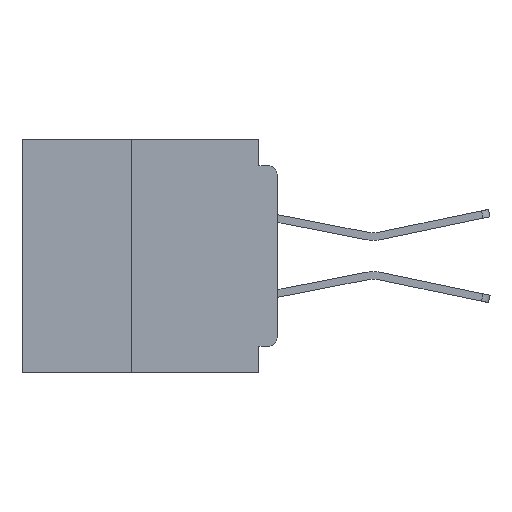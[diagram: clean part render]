
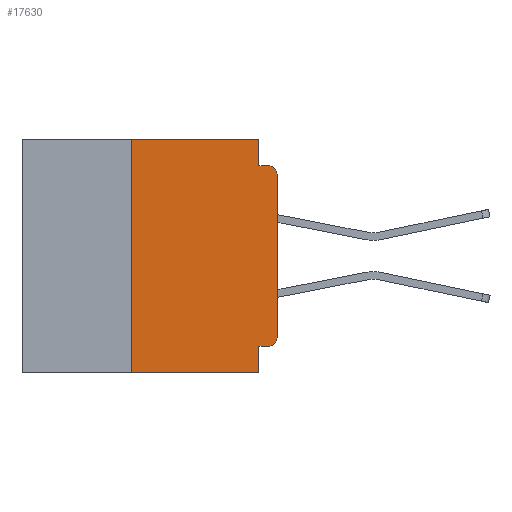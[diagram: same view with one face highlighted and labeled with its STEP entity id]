
A CAD part, left-side view. The second image highlights one B-rep face of the part: STEP entity #17630.
In plain terms, the highlighted planar face has unit normal (-1, 0, 0).
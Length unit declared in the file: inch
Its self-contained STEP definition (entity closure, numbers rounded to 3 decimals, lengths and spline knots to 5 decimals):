
#863 = VERTEX_POINT ( 'NONE', #28251 ) ;
#1961 = VERTEX_POINT ( 'NONE', #22788 ) ;
#3124 = DIRECTION ( 'NONE',  ( 0., -1., 0. ) ) ;
#4125 = DIRECTION ( 'NONE',  ( 0., 0., 1. ) ) ;
#4269 = DIRECTION ( 'NONE',  ( 0., -1., 0. ) ) ;
#4280 = ORIENTED_EDGE ( 'NONE', *, *, #34352, .F. ) ;
#4427 = VECTOR ( 'NONE', #4125, 39.37008 ) ;
#4716 = EDGE_CURVE ( 'NONE', #42640, #46882, #25046, .T. ) ;
#4944 = LINE ( 'NONE', #31945, #31008 ) ;
#5042 = DIRECTION ( 'NONE',  ( 0., 1., 0. ) ) ;
#5555 = CARTESIAN_POINT ( 'NONE',  ( 0., 0.031, -0.4 ) ) ;
#5792 = LINE ( 'NONE', #15640, #31858 ) ;
#5839 = CARTESIAN_POINT ( 'NONE',  ( 0., 0.015, -0.355 ) ) ;
#6506 = DIRECTION ( 'NONE',  ( -1., 0., 0. ) ) ;
#6541 = DIRECTION ( 'NONE',  ( 0., 0., 1. ) ) ;
#8428 = VERTEX_POINT ( 'NONE', #54226 ) ;
#10193 = DIRECTION ( 'NONE',  ( 0., 0., -1. ) ) ;
#10195 = CARTESIAN_POINT ( 'NONE',  ( 0., 0., -0.06 ) ) ;
#10734 = PLANE ( 'NONE',  #24280 ) ;
#11430 = EDGE_LOOP ( 'NONE', ( #28091, #58225, #35325, #39648, #4280, #16560, #43976, #33173, #38935, #40391 ) ) ;
#11553 = AXIS2_PLACEMENT_3D ( 'NONE', #34167, #6506, #38782 ) ;
#13358 = EDGE_CURVE ( 'NONE', #1961, #33585, #40653, .T. ) ;
#14480 = LINE ( 'NONE', #23414, #49854 ) ;
#15387 = DIRECTION ( 'NONE',  ( 1., 0., 0. ) ) ;
#15640 = CARTESIAN_POINT ( 'NONE',  ( 0., 0.25, -0.4 ) ) ;
#16560 = ORIENTED_EDGE ( 'NONE', *, *, #54841, .F. ) ;
#17630 = ADVANCED_FACE ( 'NONE', ( #53106 ), #10734, .F. ) ;
#18800 = VERTEX_POINT ( 'NONE', #10195 ) ;
#21781 = CARTESIAN_POINT ( 'NONE',  ( 0., 0.031, 0. ) ) ;
#22788 = CARTESIAN_POINT ( 'NONE',  ( 0., 0.25, -0.4 ) ) ;
#23414 = CARTESIAN_POINT ( 'NONE',  ( 0., 0., -0.355 ) ) ;
#24280 = AXIS2_PLACEMENT_3D ( 'NONE', #43015, #15387, #47653 ) ;
#24328 = VERTEX_POINT ( 'NONE', #43572 ) ;
#25046 = CIRCLE ( 'NONE', #49251, 0.015 ) ;
#26433 = DIRECTION ( 'NONE',  ( 0., 0., -1. ) ) ;
#27330 = LINE ( 'NONE', #21781, #50355 ) ;
#27472 = EDGE_CURVE ( 'NONE', #18800, #863, #30066, .T. ) ;
#28091 = ORIENTED_EDGE ( 'NONE', *, *, #36824, .T. ) ;
#28251 = CARTESIAN_POINT ( 'NONE',  ( 0., 0.015, -0.045 ) ) ;
#30066 = CIRCLE ( 'NONE', #11553, 0.015 ) ;
#30070 = CARTESIAN_POINT ( 'NONE',  ( 0., 0.031, -0.4 ) ) ;
#30413 = DIRECTION ( 'NONE',  ( 0., -1., 0. ) ) ;
#31008 = VECTOR ( 'NONE', #4269, 39.37008 ) ;
#31473 = CARTESIAN_POINT ( 'NONE',  ( 0., 0., -0.34 ) ) ;
#31858 = VECTOR ( 'NONE', #6541, 39.37008 ) ;
#31945 = CARTESIAN_POINT ( 'NONE',  ( 0., 0., -0.045 ) ) ;
#32117 = LINE ( 'NONE', #44641, #42879 ) ;
#33173 = ORIENTED_EDGE ( 'NONE', *, *, #45171, .F. ) ;
#33585 = VERTEX_POINT ( 'NONE', #30070 ) ;
#34167 = CARTESIAN_POINT ( 'NONE',  ( 0., 0.015, -0.06 ) ) ;
#34352 = EDGE_CURVE ( 'NONE', #8428, #59112, #32117, .T. ) ;
#35325 = ORIENTED_EDGE ( 'NONE', *, *, #44308, .F. ) ;
#36824 = EDGE_CURVE ( 'NONE', #46882, #18800, #41220, .T. ) ;
#38782 = DIRECTION ( 'NONE',  ( 0., 0., -1. ) ) ;
#38935 = ORIENTED_EDGE ( 'NONE', *, *, #46390, .F. ) ;
#39648 = ORIENTED_EDGE ( 'NONE', *, *, #56187, .F. ) ;
#40391 = ORIENTED_EDGE ( 'NONE', *, *, #4716, .T. ) ;
#40653 = LINE ( 'NONE', #48709, #52826 ) ;
#41220 = LINE ( 'NONE', #59187, #4427 ) ;
#42640 = VERTEX_POINT ( 'NONE', #5839 ) ;
#42879 = VECTOR ( 'NONE', #3124, 39.37008 ) ;
#43015 = CARTESIAN_POINT ( 'NONE',  ( 0., 0.437, 0. ) ) ;
#43572 = CARTESIAN_POINT ( 'NONE',  ( 0., 0.031, -0.355 ) ) ;
#43976 = ORIENTED_EDGE ( 'NONE', *, *, #13358, .T. ) ;
#44308 = EDGE_CURVE ( 'NONE', #57596, #863, #4944, .T. ) ;
#44641 = CARTESIAN_POINT ( 'NONE',  ( 0., 0.437, 0. ) ) ;
#44679 = DIRECTION ( 'NONE',  ( 0., 0., -1. ) ) ;
#44982 = DIRECTION ( 'NONE',  ( -1., 0., 0. ) ) ;
#44991 = CARTESIAN_POINT ( 'NONE',  ( 0., 0.015, -0.34 ) ) ;
#45171 = EDGE_CURVE ( 'NONE', #24328, #33585, #59219, .T. ) ;
#45771 = CARTESIAN_POINT ( 'NONE',  ( 0., 0.031, -0.045 ) ) ;
#46390 = EDGE_CURVE ( 'NONE', #42640, #24328, #14480, .T. ) ;
#46882 = VERTEX_POINT ( 'NONE', #31473 ) ;
#47112 = VECTOR ( 'NONE', #10193, 39.37008 ) ;
#47653 = DIRECTION ( 'NONE',  ( 0., 0., -1. ) ) ;
#48709 = CARTESIAN_POINT ( 'NONE',  ( 0., 0.437, -0.4 ) ) ;
#49251 = AXIS2_PLACEMENT_3D ( 'NONE', #44991, #44982, #44679 ) ;
#49854 = VECTOR ( 'NONE', #5042, 39.37008 ) ;
#50355 = VECTOR ( 'NONE', #26433, 39.37008 ) ;
#52826 = VECTOR ( 'NONE', #30413, 39.37008 ) ;
#53106 = FACE_OUTER_BOUND ( 'NONE', #11430, .T. ) ;
#54226 = CARTESIAN_POINT ( 'NONE',  ( 0., 0.25, 0. ) ) ;
#54841 = EDGE_CURVE ( 'NONE', #1961, #8428, #5792, .T. ) ;
#55578 = CARTESIAN_POINT ( 'NONE',  ( 0., 0.031, 0. ) ) ;
#56187 = EDGE_CURVE ( 'NONE', #59112, #57596, #27330, .T. ) ;
#57596 = VERTEX_POINT ( 'NONE', #45771 ) ;
#58225 = ORIENTED_EDGE ( 'NONE', *, *, #27472, .T. ) ;
#59112 = VERTEX_POINT ( 'NONE', #55578 ) ;
#59187 = CARTESIAN_POINT ( 'NONE',  ( 0., 0., 0. ) ) ;
#59219 = LINE ( 'NONE', #5555, #47112 ) ;
